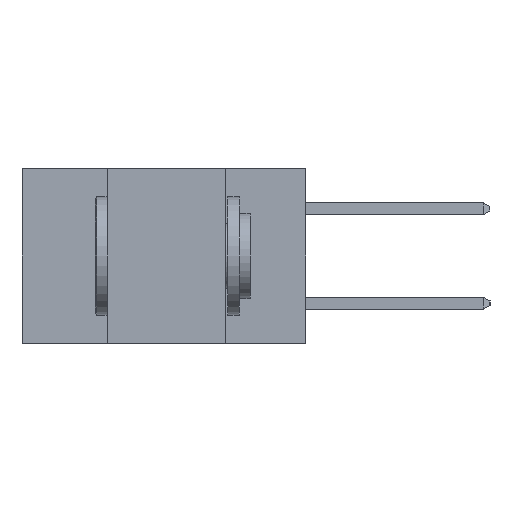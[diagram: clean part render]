
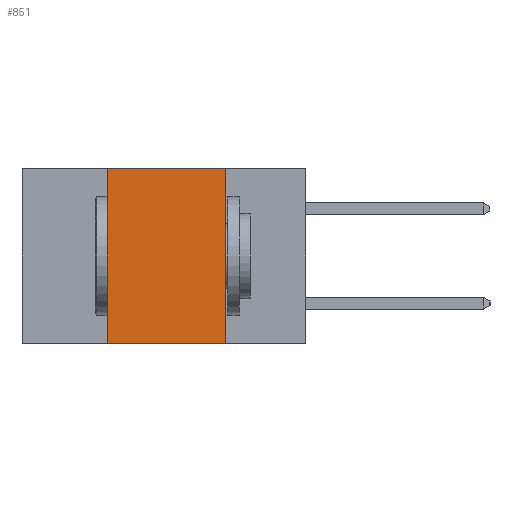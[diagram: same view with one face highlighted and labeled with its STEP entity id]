
A CAD part, left-side view. The second image highlights one B-rep face of the part: STEP entity #851.
In plain terms, the highlighted planar face has unit normal (-1, 0, 0).
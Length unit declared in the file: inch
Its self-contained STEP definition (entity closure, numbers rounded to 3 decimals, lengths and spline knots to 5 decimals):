
#851 = ADVANCED_FACE ( 'NONE', ( #7090 ), #2386, .F. ) ;
#1171 = ORIENTED_EDGE ( 'NONE', *, *, #16605, .F. ) ;
#1216 = ORIENTED_EDGE ( 'NONE', *, *, #22662, .F. ) ;
#1219 = AXIS2_PLACEMENT_3D ( 'NONE', #15861, #7539, #10545 ) ;
#1354 = ORIENTED_EDGE ( 'NONE', *, *, #17055, .F. ) ;
#1404 = ORIENTED_EDGE ( 'NONE', *, *, #22596, .T. ) ;
#1484 = DIRECTION ( 'NONE',  ( 0., 0., 1. ) ) ;
#2386 = PLANE ( 'NONE',  #1219 ) ;
#4056 = VECTOR ( 'NONE', #1484, 39.37008 ) ;
#5055 = VERTEX_POINT ( 'NONE', #12709 ) ;
#6043 = VERTEX_POINT ( 'NONE', #21437 ) ;
#6449 = DIRECTION ( 'NONE',  ( 0., -1., 0. ) ) ;
#6596 = DIRECTION ( 'NONE',  ( 0., -1., 0. ) ) ;
#7090 = FACE_OUTER_BOUND ( 'NONE', #11140, .T. ) ;
#7539 = DIRECTION ( 'NONE',  ( 1., 0., 0. ) ) ;
#9497 = VECTOR ( 'NONE', #14170, 39.37008 ) ;
#10088 = VECTOR ( 'NONE', #6596, 39.37008 ) ;
#10545 = DIRECTION ( 'NONE',  ( 0., 0., -1. ) ) ;
#11140 = EDGE_LOOP ( 'NONE', ( #1171, #1216, #1354, #1404 ) ) ;
#12335 = CARTESIAN_POINT ( 'NONE',  ( 0., 0.17, 0. ) ) ;
#12508 = VECTOR ( 'NONE', #6449, 39.37008 ) ;
#12709 = CARTESIAN_POINT ( 'NONE',  ( 0., 0.42, -0.37 ) ) ;
#12813 = CARTESIAN_POINT ( 'NONE',  ( 0., 0.17, -0.37 ) ) ;
#12830 = CARTESIAN_POINT ( 'NONE',  ( 0., 0.17, -0.37 ) ) ;
#12924 = VERTEX_POINT ( 'NONE', #12830 ) ;
#14170 = DIRECTION ( 'NONE',  ( 0., 0., -1. ) ) ;
#14696 = LINE ( 'NONE', #20439, #10088 ) ;
#15266 = CARTESIAN_POINT ( 'NONE',  ( 0., 0.6, -0.37 ) ) ;
#15861 = CARTESIAN_POINT ( 'NONE',  ( 0., 0.6, 0. ) ) ;
#16605 = EDGE_CURVE ( 'NONE', #22107, #12924, #19709, .T. ) ;
#17055 = EDGE_CURVE ( 'NONE', #5055, #6043, #22565, .T. ) ;
#19709 = LINE ( 'NONE', #12813, #9497 ) ;
#20439 = CARTESIAN_POINT ( 'NONE',  ( 0., 0.6, 0. ) ) ;
#20782 = LINE ( 'NONE', #15266, #12508 ) ;
#21437 = CARTESIAN_POINT ( 'NONE',  ( 0., 0.42, 0. ) ) ;
#22107 = VERTEX_POINT ( 'NONE', #12335 ) ;
#22430 = CARTESIAN_POINT ( 'NONE',  ( 0., 0.42, -0.37 ) ) ;
#22565 = LINE ( 'NONE', #22430, #4056 ) ;
#22596 = EDGE_CURVE ( 'NONE', #5055, #12924, #20782, .T. ) ;
#22662 = EDGE_CURVE ( 'NONE', #6043, #22107, #14696, .T. ) ;
